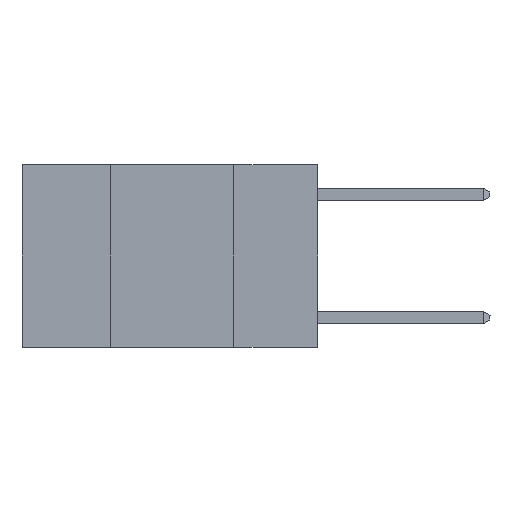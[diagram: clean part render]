
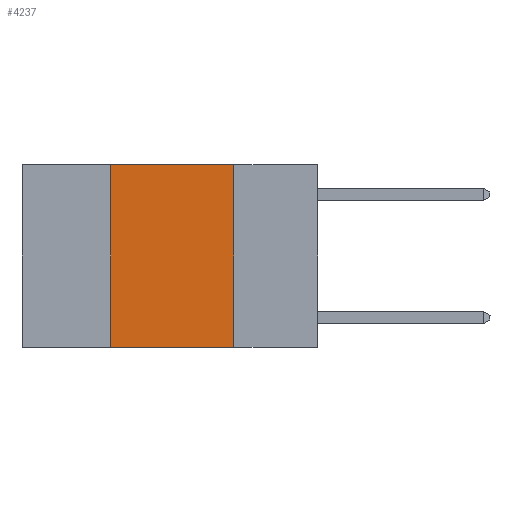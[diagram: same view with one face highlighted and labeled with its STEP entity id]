
A CAD part, left-side view. The second image highlights one B-rep face of the part: STEP entity #4237.
In plain terms, the highlighted planar face has unit normal (-1, 0, 0).
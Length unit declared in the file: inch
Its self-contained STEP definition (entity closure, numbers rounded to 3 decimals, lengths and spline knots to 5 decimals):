
#174 = CARTESIAN_POINT ( 'NONE',  ( 0., 0.6, 0. ) ) ;
#1387 = VECTOR ( 'NONE', #3600, 39.37008 ) ;
#1449 = CARTESIAN_POINT ( 'NONE',  ( 0., 0.17, -0.37 ) ) ;
#2767 = VECTOR ( 'NONE', #24567, 39.37008 ) ;
#3600 = DIRECTION ( 'NONE',  ( 0., 0., 1. ) ) ;
#4034 = DIRECTION ( 'NONE',  ( 1., 0., 0. ) ) ;
#4237 = ADVANCED_FACE ( 'NONE', ( #18516 ), #26404, .F. ) ;
#4623 = EDGE_CURVE ( 'NONE', #24634, #23657, #20960, .T. ) ;
#5749 = CARTESIAN_POINT ( 'NONE',  ( 0., 0.42, 0. ) ) ;
#5785 = ORIENTED_EDGE ( 'NONE', *, *, #15158, .F. ) ;
#5849 = VECTOR ( 'NONE', #9809, 39.37008 ) ;
#6342 = VECTOR ( 'NONE', #13848, 39.37008 ) ;
#6349 = ORIENTED_EDGE ( 'NONE', *, *, #24911, .F. ) ;
#7818 = CARTESIAN_POINT ( 'NONE',  ( 0., 0.42, 0. ) ) ;
#9809 = DIRECTION ( 'NONE',  ( 0., -1., 0. ) ) ;
#10535 = AXIS2_PLACEMENT_3D ( 'NONE', #12504, #4034, #14753 ) ;
#10744 = ORIENTED_EDGE ( 'NONE', *, *, #4623, .T. ) ;
#10771 = CARTESIAN_POINT ( 'NONE',  ( 0., 0.6, -0.37 ) ) ;
#12024 = ORIENTED_EDGE ( 'NONE', *, *, #17640, .F. ) ;
#12279 = LINE ( 'NONE', #174, #2767 ) ;
#12306 = VERTEX_POINT ( 'NONE', #7818 ) ;
#12504 = CARTESIAN_POINT ( 'NONE',  ( 0., 0.6, 0. ) ) ;
#13308 = VERTEX_POINT ( 'NONE', #18459 ) ;
#13794 = LINE ( 'NONE', #5749, #1387 ) ;
#13848 = DIRECTION ( 'NONE',  ( 0., 0., -1. ) ) ;
#13979 = CARTESIAN_POINT ( 'NONE',  ( 0., 0.17, 0. ) ) ;
#14753 = DIRECTION ( 'NONE',  ( 0., 0., -1. ) ) ;
#15158 = EDGE_CURVE ( 'NONE', #12306, #13308, #12279, .T. ) ;
#16845 = EDGE_LOOP ( 'NONE', ( #6349, #5785, #12024, #10744 ) ) ;
#17640 = EDGE_CURVE ( 'NONE', #24634, #12306, #13794, .T. ) ;
#18067 = CARTESIAN_POINT ( 'NONE',  ( 0., 0.42, -0.37 ) ) ;
#18459 = CARTESIAN_POINT ( 'NONE',  ( 0., 0.17, 0. ) ) ;
#18516 = FACE_OUTER_BOUND ( 'NONE', #16845, .T. ) ;
#20960 = LINE ( 'NONE', #10771, #5849 ) ;
#23657 = VERTEX_POINT ( 'NONE', #1449 ) ;
#23762 = LINE ( 'NONE', #13979, #6342 ) ;
#24567 = DIRECTION ( 'NONE',  ( 0., -1., 0. ) ) ;
#24634 = VERTEX_POINT ( 'NONE', #18067 ) ;
#24911 = EDGE_CURVE ( 'NONE', #13308, #23657, #23762, .T. ) ;
#26404 = PLANE ( 'NONE',  #10535 ) ;
